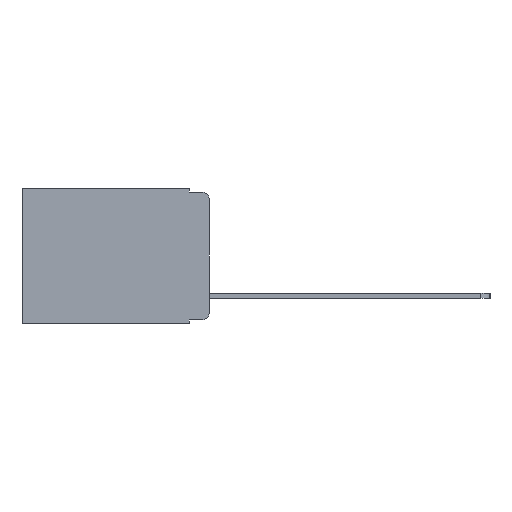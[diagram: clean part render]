
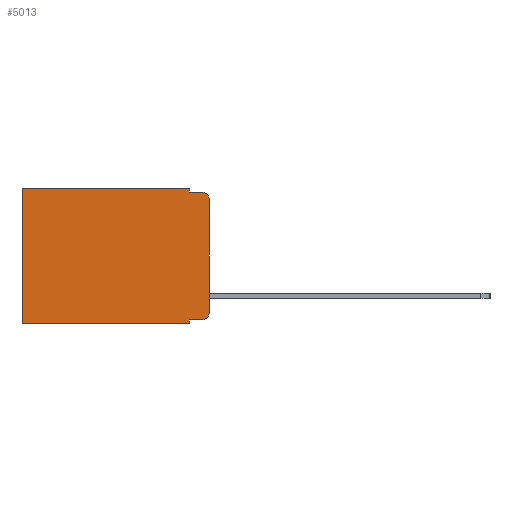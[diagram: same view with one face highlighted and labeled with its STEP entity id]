
A CAD part, left-side view. The second image highlights one B-rep face of the part: STEP entity #5013.
In plain terms, the highlighted planar face has unit normal (-1, 0, 0).
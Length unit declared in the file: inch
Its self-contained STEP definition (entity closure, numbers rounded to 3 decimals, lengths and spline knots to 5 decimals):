
#148 = EDGE_LOOP ( 'NONE', ( #4773, #4908, #5133, #5363, #5486, #5556, #5912, #6525, #6758, #6882 ) ) ;
#244 = CARTESIAN_POINT ( 'NONE',  ( 0.298, 0.051, -0.01 ) ) ;
#760 = EDGE_CURVE ( 'NONE', #4913, #5977, #13905, .T. ) ;
#895 = AXIS2_PLACEMENT_3D ( 'NONE', #6411, #7880, #17277 ) ;
#1162 = LINE ( 'NONE', #2777, #8315 ) ;
#1543 = EDGE_CURVE ( 'NONE', #15331, #5799, #9709, .T. ) ;
#1913 = CARTESIAN_POINT ( 'NONE',  ( 0.298, 0., -0.313 ) ) ;
#2011 = LINE ( 'NONE', #7993, #16246 ) ;
#2258 = AXIS2_PLACEMENT_3D ( 'NONE', #13297, #2730, #2729 ) ;
#2267 = LINE ( 'NONE', #7937, #16457 ) ;
#2729 = DIRECTION ( 'NONE',  ( 0., 0., -1. ) ) ;
#2730 = DIRECTION ( 'NONE',  ( 1., 0., 0. ) ) ;
#2777 = CARTESIAN_POINT ( 'NONE',  ( 0.298, 0.051, -0.01 ) ) ;
#2985 = EDGE_CURVE ( 'NONE', #15331, #16094, #2011, .T. ) ;
#3877 = VECTOR ( 'NONE', #8554, 39.37008 ) ;
#3878 = CARTESIAN_POINT ( 'NONE',  ( 0.298, 0.051, 0. ) ) ;
#3999 = DIRECTION ( 'NONE',  ( -1., 0., 0. ) ) ;
#4277 = CARTESIAN_POINT ( 'NONE',  ( 0.298, 0., -0.03 ) ) ;
#4773 = ORIENTED_EDGE ( 'NONE', *, *, #760, .F. ) ;
#4908 = ORIENTED_EDGE ( 'NONE', *, *, #5283, .T. ) ;
#4913 = VERTEX_POINT ( 'NONE', #4277 ) ;
#5013 = ADVANCED_FACE ( 'NONE', ( #9202 ), #8355, .F. ) ;
#5133 = ORIENTED_EDGE ( 'NONE', *, *, #16373, .F. ) ;
#5283 = EDGE_CURVE ( 'NONE', #4913, #8699, #5344, .T. ) ;
#5344 = CIRCLE ( 'NONE', #895, 0.02 ) ;
#5363 = ORIENTED_EDGE ( 'NONE', *, *, #1543, .F. ) ;
#5404 = EDGE_CURVE ( 'NONE', #7932, #13936, #14045, .T. ) ;
#5486 = ORIENTED_EDGE ( 'NONE', *, *, #2985, .T. ) ;
#5535 = DIRECTION ( 'NONE',  ( 0., 0., -1. ) ) ;
#5556 = ORIENTED_EDGE ( 'NONE', *, *, #10342, .T. ) ;
#5776 = CARTESIAN_POINT ( 'NONE',  ( 0.298, 0.473, -0.343 ) ) ;
#5799 = VERTEX_POINT ( 'NONE', #244 ) ;
#5912 = ORIENTED_EDGE ( 'NONE', *, *, #5404, .F. ) ;
#5977 = VERTEX_POINT ( 'NONE', #1913 ) ;
#6135 = VERTEX_POINT ( 'NONE', #7562 ) ;
#6298 = VECTOR ( 'NONE', #15519, 39.37008 ) ;
#6411 = CARTESIAN_POINT ( 'NONE',  ( 0.298, 0.02, -0.03 ) ) ;
#6525 = ORIENTED_EDGE ( 'NONE', *, *, #7668, .F. ) ;
#6574 = VECTOR ( 'NONE', #12444, 39.37008 ) ;
#6758 = ORIENTED_EDGE ( 'NONE', *, *, #8007, .T. ) ;
#6882 = ORIENTED_EDGE ( 'NONE', *, *, #15353, .T. ) ;
#7088 = DIRECTION ( 'NONE',  ( 0., -1., 0. ) ) ;
#7147 = LINE ( 'NONE', #13632, #7548 ) ;
#7548 = VECTOR ( 'NONE', #5535, 39.37008 ) ;
#7562 = CARTESIAN_POINT ( 'NONE',  ( 0.298, 0.051, -0.333 ) ) ;
#7668 = EDGE_CURVE ( 'NONE', #6135, #7932, #14772, .T. ) ;
#7880 = DIRECTION ( 'NONE',  ( -1., 0., 0. ) ) ;
#7932 = VERTEX_POINT ( 'NONE', #12288 ) ;
#7937 = CARTESIAN_POINT ( 'NONE',  ( 0.298, 0.051, -0.333 ) ) ;
#7993 = CARTESIAN_POINT ( 'NONE',  ( 0.298, 0., 0. ) ) ;
#8007 = EDGE_CURVE ( 'NONE', #6135, #16045, #2267, .T. ) ;
#8071 = AXIS2_PLACEMENT_3D ( 'NONE', #12210, #3999, #13569 ) ;
#8315 = VECTOR ( 'NONE', #7088, 39.37008 ) ;
#8355 = PLANE ( 'NONE',  #2258 ) ;
#8495 = CARTESIAN_POINT ( 'NONE',  ( 0.298, 0.051, 0. ) ) ;
#8554 = DIRECTION ( 'NONE',  ( 0., 0., -1. ) ) ;
#8699 = VERTEX_POINT ( 'NONE', #15928 ) ;
#9030 = CARTESIAN_POINT ( 'NONE',  ( 0.298, 0.473, 0. ) ) ;
#9202 = FACE_OUTER_BOUND ( 'NONE', #148, .T. ) ;
#9390 = DIRECTION ( 'NONE',  ( 0., 1., 0. ) ) ;
#9709 = LINE ( 'NONE', #17433, #6574 ) ;
#10342 = EDGE_CURVE ( 'NONE', #16094, #13936, #7147, .T. ) ;
#10438 = CARTESIAN_POINT ( 'NONE',  ( 0.298, 0., -0.343 ) ) ;
#10607 = DIRECTION ( 'NONE',  ( 0., -1., 0. ) ) ;
#11868 = DIRECTION ( 'NONE',  ( 0., 1., 0. ) ) ;
#12210 = CARTESIAN_POINT ( 'NONE',  ( 0.298, 0.02, -0.313 ) ) ;
#12288 = CARTESIAN_POINT ( 'NONE',  ( 0.298, 0.051, -0.343 ) ) ;
#12444 = DIRECTION ( 'NONE',  ( 0., 0., -1. ) ) ;
#13297 = CARTESIAN_POINT ( 'NONE',  ( 0.298, 0., 0. ) ) ;
#13569 = DIRECTION ( 'NONE',  ( 0., 0., -1. ) ) ;
#13632 = CARTESIAN_POINT ( 'NONE',  ( 0.298, 0.473, 0. ) ) ;
#13905 = LINE ( 'NONE', #14377, #6298 ) ;
#13936 = VERTEX_POINT ( 'NONE', #5776 ) ;
#13965 = CARTESIAN_POINT ( 'NONE',  ( 0.298, 0.02, -0.333 ) ) ;
#14045 = LINE ( 'NONE', #10438, #17170 ) ;
#14377 = CARTESIAN_POINT ( 'NONE',  ( 0.298, 0., 0. ) ) ;
#14772 = LINE ( 'NONE', #8495, #3877 ) ;
#15331 = VERTEX_POINT ( 'NONE', #3878 ) ;
#15353 = EDGE_CURVE ( 'NONE', #16045, #5977, #16148, .T. ) ;
#15519 = DIRECTION ( 'NONE',  ( 0., 0., -1. ) ) ;
#15928 = CARTESIAN_POINT ( 'NONE',  ( 0.298, 0.02, -0.01 ) ) ;
#16045 = VERTEX_POINT ( 'NONE', #13965 ) ;
#16094 = VERTEX_POINT ( 'NONE', #9030 ) ;
#16148 = CIRCLE ( 'NONE', #8071, 0.02 ) ;
#16246 = VECTOR ( 'NONE', #9390, 39.37008 ) ;
#16373 = EDGE_CURVE ( 'NONE', #5799, #8699, #1162, .T. ) ;
#16457 = VECTOR ( 'NONE', #10607, 39.37008 ) ;
#17170 = VECTOR ( 'NONE', #11868, 39.37008 ) ;
#17277 = DIRECTION ( 'NONE',  ( 0., 0., -1. ) ) ;
#17433 = CARTESIAN_POINT ( 'NONE',  ( 0.298, 0.051, 0. ) ) ;
